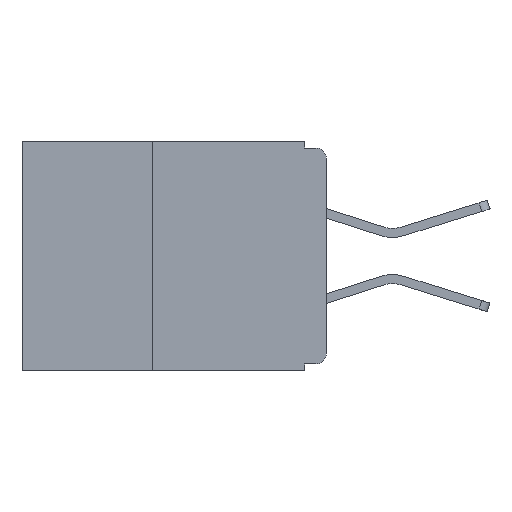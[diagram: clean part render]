
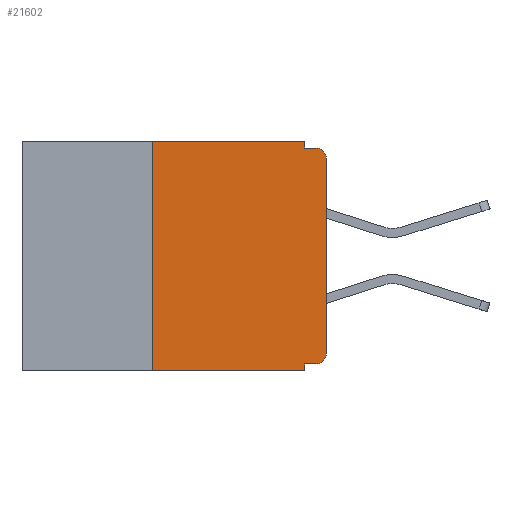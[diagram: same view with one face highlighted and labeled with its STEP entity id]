
A CAD part, left-side view. The second image highlights one B-rep face of the part: STEP entity #21602.
In plain terms, the highlighted planar face has unit normal (-1, 0, 0).
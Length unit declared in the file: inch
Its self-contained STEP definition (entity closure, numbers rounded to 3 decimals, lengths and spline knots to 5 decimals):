
#9 = CARTESIAN_POINT ( 'NONE',  ( 0., 0.031, -0.33 ) ) ;
#517 = CARTESIAN_POINT ( 'NONE',  ( 0., 0.031, 0. ) ) ;
#705 = CARTESIAN_POINT ( 'NONE',  ( 0., 0.25, -0.33 ) ) ;
#760 = CARTESIAN_POINT ( 'NONE',  ( 0., 0.437, 0. ) ) ;
#1278 = LINE ( 'NONE', #705, #10401 ) ;
#1293 = EDGE_CURVE ( 'NONE', #6377, #8072, #3810, .T. ) ;
#1573 = DIRECTION ( 'NONE',  ( 0., 0., -1. ) ) ;
#1646 = CARTESIAN_POINT ( 'NONE',  ( 0., 0.25, 0. ) ) ;
#1652 = DIRECTION ( 'NONE',  ( 0., -1., 0. ) ) ;
#1780 = ORIENTED_EDGE ( 'NONE', *, *, #12307, .T. ) ;
#2020 = ORIENTED_EDGE ( 'NONE', *, *, #1293, .T. ) ;
#2183 = VERTEX_POINT ( 'NONE', #15632 ) ;
#2354 = EDGE_CURVE ( 'NONE', #20310, #6333, #18416, .T. ) ;
#2624 = ORIENTED_EDGE ( 'NONE', *, *, #21399, .F. ) ;
#2649 = EDGE_CURVE ( 'NONE', #8072, #12249, #17088, .T. ) ;
#3440 = CARTESIAN_POINT ( 'NONE',  ( 0., 0.031, -0.01 ) ) ;
#3510 = LINE ( 'NONE', #9, #7527 ) ;
#3810 = LINE ( 'NONE', #8404, #17899 ) ;
#3951 = ORIENTED_EDGE ( 'NONE', *, *, #12873, .F. ) ;
#4618 = EDGE_LOOP ( 'NONE', ( #2020, #11937, #14827, #16139, #18269, #2624, #1780, #16712, #3951, #21907 ) ) ;
#4687 = DIRECTION ( 'NONE',  ( 1., 0., 0. ) ) ;
#4871 = CARTESIAN_POINT ( 'NONE',  ( 0., 0.031, 0. ) ) ;
#5286 = VERTEX_POINT ( 'NONE', #13805 ) ;
#5678 = VECTOR ( 'NONE', #11172, 39.37008 ) ;
#6333 = VERTEX_POINT ( 'NONE', #4871 ) ;
#6377 = VERTEX_POINT ( 'NONE', #21924 ) ;
#7281 = VECTOR ( 'NONE', #1652, 39.37008 ) ;
#7315 = EDGE_CURVE ( 'NONE', #2183, #6377, #17146, .T. ) ;
#7527 = VECTOR ( 'NONE', #18811, 39.37008 ) ;
#7806 = LINE ( 'NONE', #21939, #7281 ) ;
#8063 = LINE ( 'NONE', #12485, #20511 ) ;
#8072 = VERTEX_POINT ( 'NONE', #13825 ) ;
#8404 = CARTESIAN_POINT ( 'NONE',  ( 0., 0., 0. ) ) ;
#8493 = DIRECTION ( 'NONE',  ( -1., 0., 0. ) ) ;
#9801 = PLANE ( 'NONE',  #19137 ) ;
#10401 = VECTOR ( 'NONE', #10981, 39.37008 ) ;
#10816 = DIRECTION ( 'NONE',  ( 0., 0., -1. ) ) ;
#10981 = DIRECTION ( 'NONE',  ( 0., 0., 1. ) ) ;
#11172 = DIRECTION ( 'NONE',  ( 0., -1., 0. ) ) ;
#11411 = VERTEX_POINT ( 'NONE', #20272 ) ;
#11830 = DIRECTION ( 'NONE',  ( -1., 0., 0. ) ) ;
#11937 = ORIENTED_EDGE ( 'NONE', *, *, #2649, .T. ) ;
#12249 = VERTEX_POINT ( 'NONE', #16043 ) ;
#12307 = EDGE_CURVE ( 'NONE', #11411, #5286, #14729, .T. ) ;
#12414 = DIRECTION ( 'NONE',  ( 0., 1., 0. ) ) ;
#12485 = CARTESIAN_POINT ( 'NONE',  ( 0., 0., -0.32 ) ) ;
#12706 = DIRECTION ( 'NONE',  ( 0., -1., 0. ) ) ;
#12830 = CARTESIAN_POINT ( 'NONE',  ( 0., 0.437, -0.33 ) ) ;
#12873 = EDGE_CURVE ( 'NONE', #2183, #19932, #8063, .T. ) ;
#13301 = EDGE_CURVE ( 'NONE', #20337, #12249, #7806, .T. ) ;
#13594 = LINE ( 'NONE', #517, #17577 ) ;
#13805 = CARTESIAN_POINT ( 'NONE',  ( 0., 0.031, -0.33 ) ) ;
#13825 = CARTESIAN_POINT ( 'NONE',  ( 0., 0., -0.025 ) ) ;
#13910 = VECTOR ( 'NONE', #12706, 39.37008 ) ;
#14729 = LINE ( 'NONE', #12830, #5678 ) ;
#14827 = ORIENTED_EDGE ( 'NONE', *, *, #13301, .F. ) ;
#14873 = CARTESIAN_POINT ( 'NONE',  ( 0., 0.437, 0. ) ) ;
#15632 = CARTESIAN_POINT ( 'NONE',  ( 0., 0.015, -0.32 ) ) ;
#16043 = CARTESIAN_POINT ( 'NONE',  ( 0., 0.015, -0.01 ) ) ;
#16139 = ORIENTED_EDGE ( 'NONE', *, *, #17269, .F. ) ;
#16400 = EDGE_CURVE ( 'NONE', #19932, #5286, #3510, .T. ) ;
#16584 = DIRECTION ( 'NONE',  ( 0., 0., -1. ) ) ;
#16712 = ORIENTED_EDGE ( 'NONE', *, *, #16400, .F. ) ;
#17088 = CIRCLE ( 'NONE', #20808, 0.015 ) ;
#17146 = CIRCLE ( 'NONE', #18023, 0.015 ) ;
#17269 = EDGE_CURVE ( 'NONE', #6333, #20337, #13594, .T. ) ;
#17577 = VECTOR ( 'NONE', #10816, 39.37008 ) ;
#17899 = VECTOR ( 'NONE', #20217, 39.37008 ) ;
#18023 = AXIS2_PLACEMENT_3D ( 'NONE', #21870, #11830, #1573 ) ;
#18269 = ORIENTED_EDGE ( 'NONE', *, *, #2354, .F. ) ;
#18416 = LINE ( 'NONE', #760, #13910 ) ;
#18630 = CARTESIAN_POINT ( 'NONE',  ( 0., 0.015, -0.025 ) ) ;
#18811 = DIRECTION ( 'NONE',  ( 0., 0., -1. ) ) ;
#19097 = FACE_OUTER_BOUND ( 'NONE', #4618, .T. ) ;
#19137 = AXIS2_PLACEMENT_3D ( 'NONE', #14873, #4687, #16584 ) ;
#19495 = CARTESIAN_POINT ( 'NONE',  ( 0., 0.031, -0.32 ) ) ;
#19932 = VERTEX_POINT ( 'NONE', #19495 ) ;
#20217 = DIRECTION ( 'NONE',  ( 0., 0., 1. ) ) ;
#20272 = CARTESIAN_POINT ( 'NONE',  ( 0., 0.25, -0.33 ) ) ;
#20310 = VERTEX_POINT ( 'NONE', #1646 ) ;
#20317 = DIRECTION ( 'NONE',  ( 0., 0., -1. ) ) ;
#20337 = VERTEX_POINT ( 'NONE', #3440 ) ;
#20511 = VECTOR ( 'NONE', #12414, 39.37008 ) ;
#20808 = AXIS2_PLACEMENT_3D ( 'NONE', #18630, #8493, #20317 ) ;
#21399 = EDGE_CURVE ( 'NONE', #11411, #20310, #1278, .T. ) ;
#21602 = ADVANCED_FACE ( 'NONE', ( #19097 ), #9801, .F. ) ;
#21870 = CARTESIAN_POINT ( 'NONE',  ( 0., 0.015, -0.305 ) ) ;
#21907 = ORIENTED_EDGE ( 'NONE', *, *, #7315, .T. ) ;
#21924 = CARTESIAN_POINT ( 'NONE',  ( 0., 0., -0.305 ) ) ;
#21939 = CARTESIAN_POINT ( 'NONE',  ( 0., 0., -0.01 ) ) ;
